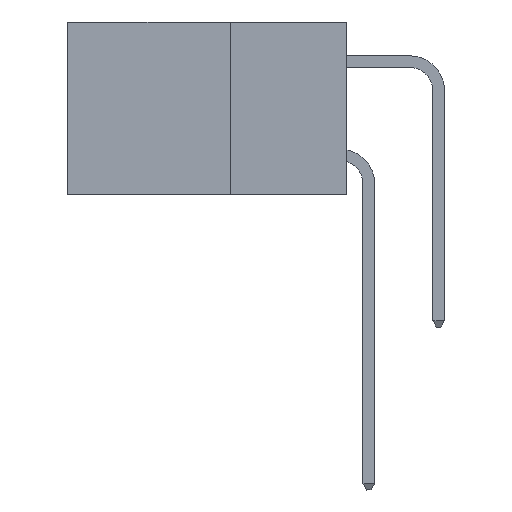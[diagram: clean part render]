
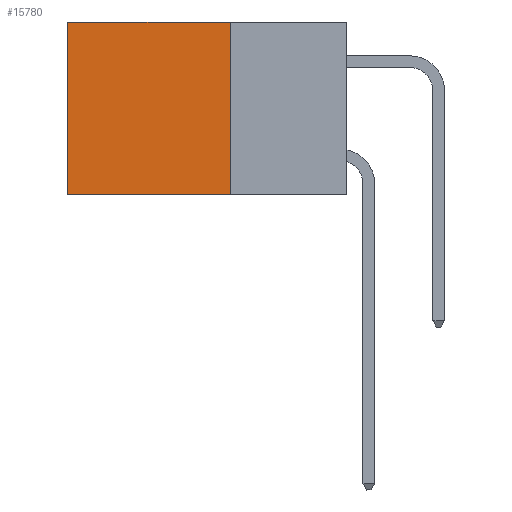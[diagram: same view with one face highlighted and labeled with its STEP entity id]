
A CAD part, left-side view. The second image highlights one B-rep face of the part: STEP entity #15780.
In plain terms, the highlighted planar face has unit normal (-1, 0, 0).
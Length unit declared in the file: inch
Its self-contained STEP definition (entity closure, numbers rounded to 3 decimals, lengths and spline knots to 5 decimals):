
#487 = EDGE_CURVE ( 'NONE', #12571, #18933, #7908, .T. ) ;
#719 = VERTEX_POINT ( 'NONE', #20243 ) ;
#1409 = VECTOR ( 'NONE', #15497, 39.37008 ) ;
#3958 = EDGE_LOOP ( 'NONE', ( #4594, #11401, #13197, #7381 ) ) ;
#4184 = VECTOR ( 'NONE', #24955, 39.37008 ) ;
#4594 = ORIENTED_EDGE ( 'NONE', *, *, #5856, .T. ) ;
#5856 = EDGE_CURVE ( 'NONE', #18933, #719, #21526, .T. ) ;
#7381 = ORIENTED_EDGE ( 'NONE', *, *, #487, .T. ) ;
#7908 = LINE ( 'NONE', #17425, #12647 ) ;
#8371 = VERTEX_POINT ( 'NONE', #17670 ) ;
#9517 = DIRECTION ( 'NONE',  ( 0., 1., 0. ) ) ;
#9576 = VECTOR ( 'NONE', #24296, 39.37008 ) ;
#10108 = CARTESIAN_POINT ( 'NONE',  ( 0.2875, 0.6, 0. ) ) ;
#11401 = ORIENTED_EDGE ( 'NONE', *, *, #18712, .F. ) ;
#11808 = PLANE ( 'NONE',  #16012 ) ;
#12338 = FACE_OUTER_BOUND ( 'NONE', #3958, .T. ) ;
#12571 = VERTEX_POINT ( 'NONE', #25612 ) ;
#12647 = VECTOR ( 'NONE', #9517, 39.37008 ) ;
#13197 = ORIENTED_EDGE ( 'NONE', *, *, #14655, .F. ) ;
#13557 = CARTESIAN_POINT ( 'NONE',  ( 0.2875, 0.25, -0.37 ) ) ;
#13875 = DIRECTION ( 'NONE',  ( 1., 0., 0. ) ) ;
#14655 = EDGE_CURVE ( 'NONE', #12571, #8371, #19309, .T. ) ;
#15497 = DIRECTION ( 'NONE',  ( 0., 1., 0. ) ) ;
#15780 = ADVANCED_FACE ( 'NONE', ( #12338 ), #11808, .F. ) ;
#16012 = AXIS2_PLACEMENT_3D ( 'NONE', #16082, #13875, #17938 ) ;
#16082 = CARTESIAN_POINT ( 'NONE',  ( 0.2875, 0.25, 0. ) ) ;
#17425 = CARTESIAN_POINT ( 'NONE',  ( 0.2875, 0.25, 0. ) ) ;
#17670 = CARTESIAN_POINT ( 'NONE',  ( 0.2875, 0.25, -0.37 ) ) ;
#17938 = DIRECTION ( 'NONE',  ( 0., 0., -1. ) ) ;
#18660 = CARTESIAN_POINT ( 'NONE',  ( 0.2875, 0.6, 0. ) ) ;
#18712 = EDGE_CURVE ( 'NONE', #8371, #719, #25655, .T. ) ;
#18933 = VERTEX_POINT ( 'NONE', #10108 ) ;
#19309 = LINE ( 'NONE', #25120, #4184 ) ;
#20243 = CARTESIAN_POINT ( 'NONE',  ( 0.2875, 0.6, -0.37 ) ) ;
#21526 = LINE ( 'NONE', #18660, #9576 ) ;
#24296 = DIRECTION ( 'NONE',  ( 0., 0., -1. ) ) ;
#24955 = DIRECTION ( 'NONE',  ( 0., 0., -1. ) ) ;
#25120 = CARTESIAN_POINT ( 'NONE',  ( 0.2875, 0.25, 0. ) ) ;
#25612 = CARTESIAN_POINT ( 'NONE',  ( 0.2875, 0.25, 0. ) ) ;
#25655 = LINE ( 'NONE', #13557, #1409 ) ;
